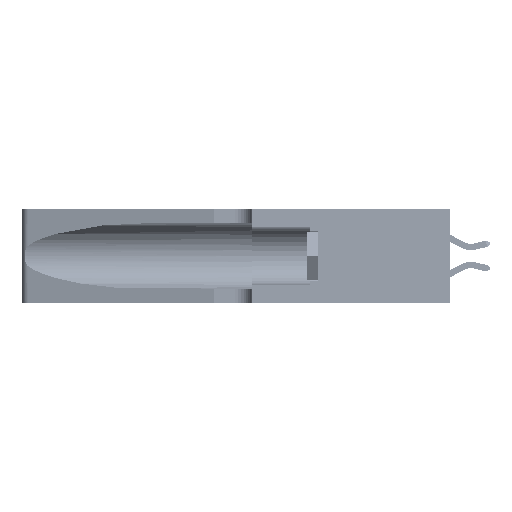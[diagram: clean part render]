
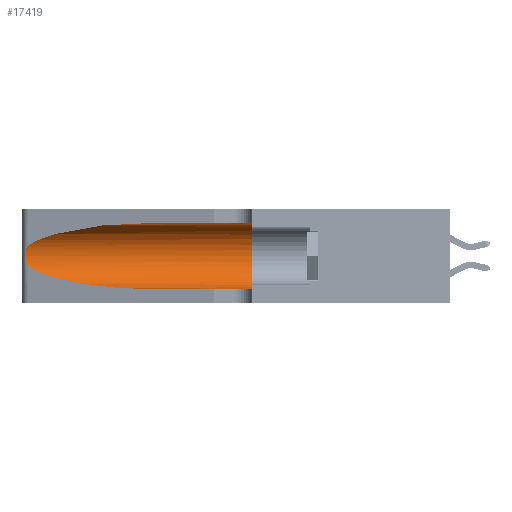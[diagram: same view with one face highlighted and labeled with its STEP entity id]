
A CAD part, left-side view. The second image highlights one B-rep face of the part: STEP entity #17419.
In plain terms, the highlighted cylindrical face has radius 3.308 mm (diameter 6.617 mm), a partial arc.
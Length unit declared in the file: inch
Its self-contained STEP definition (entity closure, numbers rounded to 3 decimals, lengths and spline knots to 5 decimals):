
#1673 = CARTESIAN_POINT ( 'NONE',  ( 0.25555, 1.22994, 0.2215 ) ) ;
#1844 = CARTESIAN_POINT ( 'NONE',  ( 0.25555, 1.22993, 0.14849 ) ) ;
#3146 = LINE ( 'NONE', #6265, #23200 ) ;
#4060 = CARTESIAN_POINT ( 'NONE',  ( 0.18966, 0.96281, 0.31525 ) ) ;
#4112 = CIRCLE ( 'NONE', #36711, 0.13025 ) ;
#5003 = CARTESIAN_POINT ( 'NONE',  ( 0.25487, 1.22718, 0.14631 ) ) ;
#5337 = CARTESIAN_POINT ( 'NONE',  ( 0.1305, 0.35, 0.31525 ) ) ;
#5390 = EDGE_CURVE ( 'NONE', #21782, #5674, #23513, .T. ) ;
#5674 = VERTEX_POINT ( 'NONE', #39478 ) ;
#5716 = CARTESIAN_POINT ( 'NONE',  ( 0.25639, 1.23184, 0.21858 ) ) ;
#6183 = EDGE_CURVE ( 'NONE', #50918, #41173, #4112, .T. ) ;
#6265 = CARTESIAN_POINT ( 'NONE',  ( 0.1305, 1.61858, 0.31525 ) ) ;
#6278 = FACE_OUTER_BOUND ( 'NONE', #45000, .T. ) ;
#6418 = EDGE_CURVE ( 'NONE', #29863, #21782, #25821, .T. ) ;
#8332 = CARTESIAN_POINT ( 'NONE',  ( 0.1305, 0.72297, 0.31525 ) ) ;
#9367 = VECTOR ( 'NONE', #33217, 39.37008 ) ;
#9411 = CARTESIAN_POINT ( 'NONE',  ( 0.1305, 0.72297, 0.05475 ) ) ;
#9772 = CARTESIAN_POINT ( 'NONE',  ( 0.25787, 1.23484, 0.2124 ) ) ;
#10321 = DIRECTION ( 'NONE',  ( 0., -1., 0. ) ) ;
#10815 = ORIENTED_EDGE ( 'NONE', *, *, #6183, .F. ) ;
#12139 = CARTESIAN_POINT ( 'NONE',  ( 0.25487, 1.22718, 0.22369 ) ) ;
#12578 = AXIS2_PLACEMENT_3D ( 'NONE', #21400, #49317, #25250 ) ;
#13795 = CARTESIAN_POINT ( 'NONE',  ( 0.26018, 1.23835, 0.19895 ) ) ;
#15693 = CYLINDRICAL_SURFACE ( 'NONE', #12578, 0.13025 ) ;
#17123 = CARTESIAN_POINT ( 'NONE',  ( 0.18966, 0.96281, 0.05475 ) ) ;
#17419 = ADVANCED_FACE ( 'NONE', ( #6278 ), #15693, .F. ) ;
#17829 = CARTESIAN_POINT ( 'NONE',  ( 0.26075, 1.23896, 0.178 ) ) ;
#18094 = EDGE_CURVE ( 'NONE', #21507, #41173, #41282, .T. ) ;
#21400 = CARTESIAN_POINT ( 'NONE',  ( 0.1305, 1.61858, 0.185 ) ) ;
#21507 = VERTEX_POINT ( 'NONE', #9411 ) ;
#21665 = CARTESIAN_POINT ( 'NONE',  ( 0.25487, 1.22718, 0.22369 ) ) ;
#21782 = VERTEX_POINT ( 'NONE', #23010 ) ;
#21837 = CARTESIAN_POINT ( 'NONE',  ( 0.25856, 1.23593, 0.16098 ) ) ;
#22814 = CARTESIAN_POINT ( 'NONE',  ( 0.1305, 0.35, 0.185 ) ) ;
#23010 = CARTESIAN_POINT ( 'NONE',  ( 0.25487, 1.22718, 0.22369 ) ) ;
#23200 = VECTOR ( 'NONE', #10321, 39.37008 ) ;
#23513 = B_SPLINE_CURVE_WITH_KNOTS ( 'NONE', 3,
 ( #21665, #1673, #5716, #9772, #37746, #13795, #41778, #17829, #45759, #21837, #49748, #25858, #1844, #29859 ),
 .UNSPECIFIED., .F., .F.,
 ( 4, 2, 2, 2, 2, 2, 4 ),
 ( 0., 0.00027, 0.00053, 0.00107, 0.0016, 0.00187, 0.00214 ),
 .UNSPECIFIED. ) ;
#25201 = ORIENTED_EDGE ( 'NONE', *, *, #5390, .T. ) ;
#25250 = DIRECTION ( 'NONE',  ( 0., 0., -1. ) ) ;
#25821 =( BOUNDED_CURVE ( )  B_SPLINE_CURVE ( 3, ( #32065, #4060, #36111, #12139 ),
 .UNSPECIFIED., .F., .F. ) 
 B_SPLINE_CURVE_WITH_KNOTS ( ( 4, 4 ),
 ( 1.5708, 2.84003 ),
 .UNSPECIFIED. ) 
 CURVE ( )  GEOMETRIC_REPRESENTATION_ITEM ( )  RATIONAL_B_SPLINE_CURVE ( ( 1., 0.87, 0.87, 1. ) ) 
 REPRESENTATION_ITEM ( '' )  );
#25858 = CARTESIAN_POINT ( 'NONE',  ( 0.25639, 1.23186, 0.15144 ) ) ;
#26842 = DIRECTION ( 'NONE',  ( 0., 0., 1. ) ) ;
#29191 = CARTESIAN_POINT ( 'NONE',  ( 0.1305, 1.61858, 0.05475 ) ) ;
#29304 = EDGE_CURVE ( 'NONE', #5674, #21507, #47491, .T. ) ;
#29859 = CARTESIAN_POINT ( 'NONE',  ( 0.25487, 1.22718, 0.14631 ) ) ;
#29863 = VERTEX_POINT ( 'NONE', #8332 ) ;
#30827 = ORIENTED_EDGE ( 'NONE', *, *, #6418, .T. ) ;
#32065 = CARTESIAN_POINT ( 'NONE',  ( 0.1305, 0.72297, 0.31525 ) ) ;
#33217 = DIRECTION ( 'NONE',  ( 0., -1., 0. ) ) ;
#33270 = ORIENTED_EDGE ( 'NONE', *, *, #18094, .T. ) ;
#34150 = EDGE_CURVE ( 'NONE', #29863, #50918, #3146, .T. ) ;
#34359 = ORIENTED_EDGE ( 'NONE', *, *, #29304, .T. ) ;
#36111 = CARTESIAN_POINT ( 'NONE',  ( 0.2373, 1.15595, 0.28018 ) ) ;
#36711 = AXIS2_PLACEMENT_3D ( 'NONE', #22814, #50716, #26842 ) ;
#37058 = CARTESIAN_POINT ( 'NONE',  ( 0.2373, 1.15595, 0.08982 ) ) ;
#37746 = CARTESIAN_POINT ( 'NONE',  ( 0.25854, 1.2359, 0.20912 ) ) ;
#39478 = CARTESIAN_POINT ( 'NONE',  ( 0.25487, 1.22718, 0.14631 ) ) ;
#41173 = VERTEX_POINT ( 'NONE', #51478 ) ;
#41282 = LINE ( 'NONE', #29191, #9367 ) ;
#41778 = CARTESIAN_POINT ( 'NONE',  ( 0.26075, 1.23896, 0.19203 ) ) ;
#45000 = EDGE_LOOP ( 'NONE', ( #30827, #25201, #34359, #33270, #10815, #51020 ) ) ;
#45082 = CARTESIAN_POINT ( 'NONE',  ( 0.1305, 0.72297, 0.05475 ) ) ;
#45759 = CARTESIAN_POINT ( 'NONE',  ( 0.26017, 1.23833, 0.17102 ) ) ;
#47491 =( BOUNDED_CURVE ( )  B_SPLINE_CURVE ( 3, ( #5003, #37058, #17123, #45082 ),
 .UNSPECIFIED., .F., .F. ) 
 B_SPLINE_CURVE_WITH_KNOTS ( ( 4, 4 ),
 ( 3.44316, 4.71239 ),
 .UNSPECIFIED. ) 
 CURVE ( )  GEOMETRIC_REPRESENTATION_ITEM ( )  RATIONAL_B_SPLINE_CURVE ( ( 1., 0.87, 0.87, 1. ) ) 
 REPRESENTATION_ITEM ( '' )  );
#49317 = DIRECTION ( 'NONE',  ( 0., -1., 0. ) ) ;
#49748 = CARTESIAN_POINT ( 'NONE',  ( 0.25789, 1.23486, 0.15765 ) ) ;
#50716 = DIRECTION ( 'NONE',  ( 0., 1., 0. ) ) ;
#50918 = VERTEX_POINT ( 'NONE', #5337 ) ;
#51020 = ORIENTED_EDGE ( 'NONE', *, *, #34150, .F. ) ;
#51478 = CARTESIAN_POINT ( 'NONE',  ( 0.1305, 0.35, 0.05475 ) ) ;
